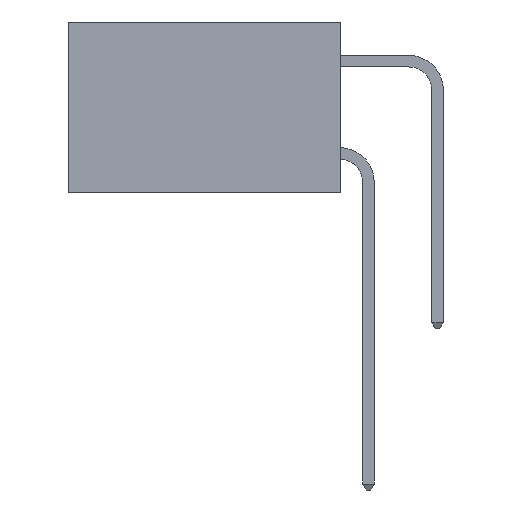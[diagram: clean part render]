
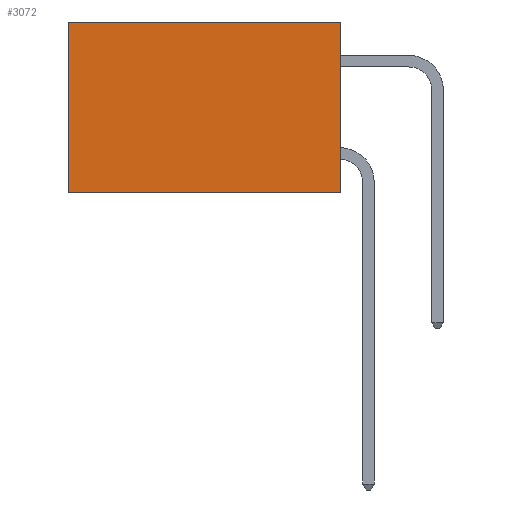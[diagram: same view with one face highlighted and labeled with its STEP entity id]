
A CAD part, left-side view. The second image highlights one B-rep face of the part: STEP entity #3072.
In plain terms, the highlighted planar face has unit normal (-1, 0, 0).
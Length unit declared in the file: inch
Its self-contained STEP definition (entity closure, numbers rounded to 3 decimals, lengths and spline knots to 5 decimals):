
#71 = VERTEX_POINT ( 'NONE', #5323 ) ;
#323 = CARTESIAN_POINT ( 'NONE',  ( 0.277, 0., -0.37 ) ) ;
#773 = VECTOR ( 'NONE', #4542, 39.37008 ) ;
#1403 = EDGE_CURVE ( 'NONE', #8525, #71, #12778, .T. ) ;
#1669 = LINE ( 'NONE', #323, #12456 ) ;
#2194 = ORIENTED_EDGE ( 'NONE', *, *, #8521, .T. ) ;
#2217 = EDGE_CURVE ( 'NONE', #10192, #71, #1669, .T. ) ;
#2380 = DIRECTION ( 'NONE',  ( 1., 0., 0. ) ) ;
#2468 = PLANE ( 'NONE',  #5991 ) ;
#2492 = FACE_OUTER_BOUND ( 'NONE', #2637, .T. ) ;
#2601 = CARTESIAN_POINT ( 'NONE',  ( 0.277, 0., -0.37 ) ) ;
#2637 = EDGE_LOOP ( 'NONE', ( #4024, #6883, #10318, #2194 ) ) ;
#3072 = ADVANCED_FACE ( 'NONE', ( #2492 ), #2468, .F. ) ;
#3276 = CARTESIAN_POINT ( 'NONE',  ( 0.277, 0., 0. ) ) ;
#3474 = CARTESIAN_POINT ( 'NONE',  ( 0.277, 0., 0. ) ) ;
#3586 = CARTESIAN_POINT ( 'NONE',  ( 0.277, 0., -0.37 ) ) ;
#3747 = DIRECTION ( 'NONE',  ( 0., 0., -1. ) ) ;
#4024 = ORIENTED_EDGE ( 'NONE', *, *, #1403, .T. ) ;
#4161 = LINE ( 'NONE', #10558, #9517 ) ;
#4542 = DIRECTION ( 'NONE',  ( 0., 1., 0. ) ) ;
#5323 = CARTESIAN_POINT ( 'NONE',  ( 0.277, 0.59, -0.37 ) ) ;
#5991 = AXIS2_PLACEMENT_3D ( 'NONE', #3586, #2380, #3747 ) ;
#6883 = ORIENTED_EDGE ( 'NONE', *, *, #2217, .F. ) ;
#7310 = VERTEX_POINT ( 'NONE', #3276 ) ;
#7409 = VECTOR ( 'NONE', #10147, 39.37008 ) ;
#8226 = EDGE_CURVE ( 'NONE', #7310, #10192, #4161, .T. ) ;
#8521 = EDGE_CURVE ( 'NONE', #7310, #8525, #9346, .T. ) ;
#8525 = VERTEX_POINT ( 'NONE', #10852 ) ;
#9346 = LINE ( 'NONE', #3474, #773 ) ;
#9517 = VECTOR ( 'NONE', #9552, 39.37008 ) ;
#9552 = DIRECTION ( 'NONE',  ( 0., 0., -1. ) ) ;
#9566 = CARTESIAN_POINT ( 'NONE',  ( 0.277, 0.59, -0.37 ) ) ;
#10147 = DIRECTION ( 'NONE',  ( 0., 0., -1. ) ) ;
#10192 = VERTEX_POINT ( 'NONE', #2601 ) ;
#10318 = ORIENTED_EDGE ( 'NONE', *, *, #8226, .F. ) ;
#10558 = CARTESIAN_POINT ( 'NONE',  ( 0.277, 0., -0.37 ) ) ;
#10852 = CARTESIAN_POINT ( 'NONE',  ( 0.277, 0.59, 0. ) ) ;
#11670 = DIRECTION ( 'NONE',  ( 0., 1., 0. ) ) ;
#12456 = VECTOR ( 'NONE', #11670, 39.37008 ) ;
#12778 = LINE ( 'NONE', #9566, #7409 ) ;
